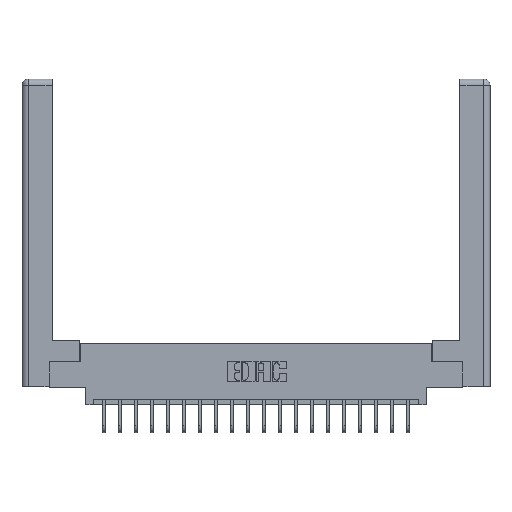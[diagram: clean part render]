
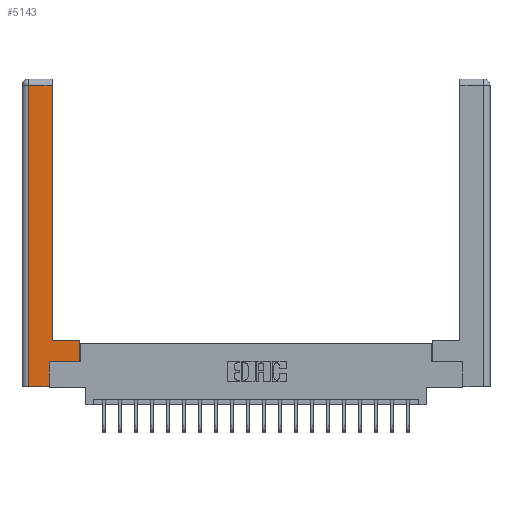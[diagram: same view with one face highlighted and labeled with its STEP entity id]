
A CAD part, top view. The second image highlights one B-rep face of the part: STEP entity #5143.
In plain terms, the highlighted planar face has unit normal (0, 0, 1).
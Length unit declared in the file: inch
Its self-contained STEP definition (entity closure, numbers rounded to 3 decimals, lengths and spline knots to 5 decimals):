
#71 = ORIENTED_EDGE ( 'NONE', *, *, #13377, .T. ) ;
#490 = DIRECTION ( 'NONE',  ( 1., 0., 0. ) ) ;
#1185 = VECTOR ( 'NONE', #15539, 39.37008 ) ;
#1858 = CARTESIAN_POINT ( 'NONE',  ( 0.0615, 0., 0. ) ) ;
#2117 = LINE ( 'NONE', #7940, #18470 ) ;
#2412 = LINE ( 'NONE', #12443, #20698 ) ;
#2569 = ORIENTED_EDGE ( 'NONE', *, *, #6428, .T. ) ;
#2645 = ORIENTED_EDGE ( 'NONE', *, *, #13858, .T. ) ;
#3815 = DIRECTION ( 'NONE',  ( 0., 1., 0. ) ) ;
#4177 = VERTEX_POINT ( 'NONE', #14943 ) ;
#4289 = ORIENTED_EDGE ( 'NONE', *, *, #11163, .T. ) ;
#4724 = CARTESIAN_POINT ( 'NONE',  ( 0., 0., 0. ) ) ;
#5059 = VERTEX_POINT ( 'NONE', #9061 ) ;
#5143 = ADVANCED_FACE ( 'NONE', ( #6737 ), #15317, .F. ) ;
#5256 = DIRECTION ( 'NONE',  ( 0., 1., 0. ) ) ;
#5641 = CARTESIAN_POINT ( 'NONE',  ( 0.0615, 2.94, 0. ) ) ;
#5762 = CARTESIAN_POINT ( 'NONE',  ( 0.565, 0.245, 0. ) ) ;
#6226 = DIRECTION ( 'NONE',  ( 0., -1., 0. ) ) ;
#6407 = CARTESIAN_POINT ( 'NONE',  ( 0.295, 0.45, 0. ) ) ;
#6428 = EDGE_CURVE ( 'NONE', #18044, #12541, #11366, .T. ) ;
#6501 = DIRECTION ( 'NONE',  ( 0., 0., -1. ) ) ;
#6640 = CARTESIAN_POINT ( 'NONE',  ( 0.565, 0.245, 0. ) ) ;
#6667 = VECTOR ( 'NONE', #17238, 39.37008 ) ;
#6737 = FACE_OUTER_BOUND ( 'NONE', #9118, .T. ) ;
#7940 = CARTESIAN_POINT ( 'NONE',  ( 0.0615, 0., 0. ) ) ;
#8079 = VECTOR ( 'NONE', #490, 39.37008 ) ;
#8191 = AXIS2_PLACEMENT_3D ( 'NONE', #4724, #6501, #18932 ) ;
#8701 = EDGE_CURVE ( 'NONE', #22159, #21526, #2117, .T. ) ;
#9061 = CARTESIAN_POINT ( 'NONE',  ( 0.295, 2.94, 0. ) ) ;
#9063 = CARTESIAN_POINT ( 'NONE',  ( 0.265, 0.245, 0. ) ) ;
#9118 = EDGE_LOOP ( 'NONE', ( #16097, #9582, #11055, #2645, #71, #2569, #14003, #4289 ) ) ;
#9582 = ORIENTED_EDGE ( 'NONE', *, *, #22360, .T. ) ;
#9786 = CARTESIAN_POINT ( 'NONE',  ( 0.295, 3., 0. ) ) ;
#9999 = LINE ( 'NONE', #9786, #1185 ) ;
#10121 = CARTESIAN_POINT ( 'NONE',  ( 0.265, 0., 0. ) ) ;
#10409 = VECTOR ( 'NONE', #12116, 39.37008 ) ;
#10588 = CARTESIAN_POINT ( 'NONE',  ( 0.265, 0., 0. ) ) ;
#10897 = EDGE_CURVE ( 'NONE', #12541, #4177, #2412, .T. ) ;
#11055 = ORIENTED_EDGE ( 'NONE', *, *, #8701, .T. ) ;
#11163 = EDGE_CURVE ( 'NONE', #4177, #14305, #19855, .T. ) ;
#11366 = LINE ( 'NONE', #6640, #6667 ) ;
#12116 = DIRECTION ( 'NONE',  ( -1., 0., 0. ) ) ;
#12443 = CARTESIAN_POINT ( 'NONE',  ( 0.565, 0.45, 0. ) ) ;
#12541 = VERTEX_POINT ( 'NONE', #5762 ) ;
#12643 = CARTESIAN_POINT ( 'NONE',  ( 0.0615, 2.94, 0. ) ) ;
#12768 = LINE ( 'NONE', #10588, #8079 ) ;
#13377 = EDGE_CURVE ( 'NONE', #15177, #18044, #16402, .T. ) ;
#13858 = EDGE_CURVE ( 'NONE', #21526, #15177, #12768, .T. ) ;
#14003 = ORIENTED_EDGE ( 'NONE', *, *, #10897, .T. ) ;
#14305 = VERTEX_POINT ( 'NONE', #6407 ) ;
#14943 = CARTESIAN_POINT ( 'NONE',  ( 0.565, 0.45, 0. ) ) ;
#15177 = VERTEX_POINT ( 'NONE', #10121 ) ;
#15317 = PLANE ( 'NONE',  #8191 ) ;
#15439 = CARTESIAN_POINT ( 'NONE',  ( 0.295, 0.45, 0. ) ) ;
#15539 = DIRECTION ( 'NONE',  ( 0., 1., 0. ) ) ;
#16097 = ORIENTED_EDGE ( 'NONE', *, *, #22302, .T. ) ;
#16402 = LINE ( 'NONE', #9063, #18657 ) ;
#17238 = DIRECTION ( 'NONE',  ( 1., 0., 0. ) ) ;
#18044 = VERTEX_POINT ( 'NONE', #18501 ) ;
#18470 = VECTOR ( 'NONE', #6226, 39.37008 ) ;
#18501 = CARTESIAN_POINT ( 'NONE',  ( 0.265, 0.245, 0. ) ) ;
#18657 = VECTOR ( 'NONE', #3815, 39.37008 ) ;
#18932 = DIRECTION ( 'NONE',  ( -1., 0., 0. ) ) ;
#19855 = LINE ( 'NONE', #15439, #10409 ) ;
#19890 = DIRECTION ( 'NONE',  ( -1., 0., 0. ) ) ;
#20698 = VECTOR ( 'NONE', #5256, 39.37008 ) ;
#20837 = VECTOR ( 'NONE', #19890, 39.37008 ) ;
#21526 = VERTEX_POINT ( 'NONE', #1858 ) ;
#22159 = VERTEX_POINT ( 'NONE', #12643 ) ;
#22302 = EDGE_CURVE ( 'NONE', #14305, #5059, #9999, .T. ) ;
#22360 = EDGE_CURVE ( 'NONE', #5059, #22159, #22501, .T. ) ;
#22501 = LINE ( 'NONE', #5641, #20837 ) ;
